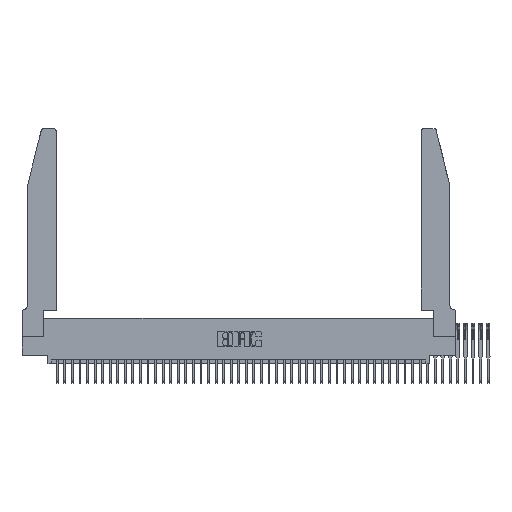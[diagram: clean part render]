
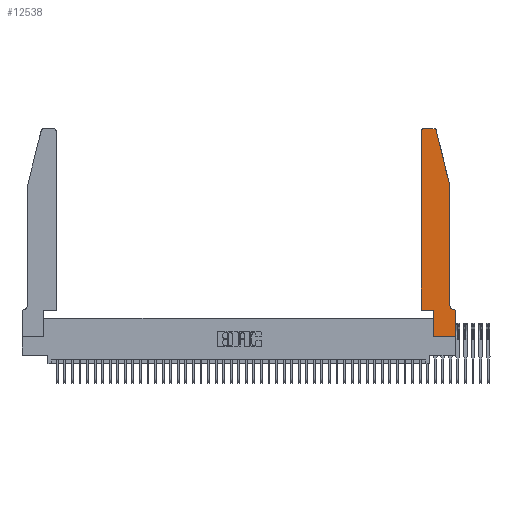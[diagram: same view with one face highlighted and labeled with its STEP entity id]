
A CAD part, top view. The second image highlights one B-rep face of the part: STEP entity #12538.
In plain terms, the highlighted face is planar.
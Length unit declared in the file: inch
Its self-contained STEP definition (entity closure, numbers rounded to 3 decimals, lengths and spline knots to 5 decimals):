
#137 = LINE ( 'NONE', #8807, #24539 ) ;
#570 = EDGE_CURVE ( 'NONE', #32551, #26741, #822, .T. ) ;
#822 = CIRCLE ( 'NONE', #26208, 0.03 ) ;
#879 = ORIENTED_EDGE ( 'NONE', *, *, #991, .F. ) ;
#991 = EDGE_CURVE ( 'NONE', #1038, #39043, #26149, .T. ) ;
#1038 = VERTEX_POINT ( 'NONE', #5005 ) ;
#1140 = LINE ( 'NONE', #37753, #32993 ) ;
#1830 = LINE ( 'NONE', #24609, #24405 ) ;
#2118 = ORIENTED_EDGE ( 'NONE', *, *, #23229, .T. ) ;
#2352 = VECTOR ( 'NONE', #24410, 39.37008 ) ;
#3321 = FACE_OUTER_BOUND ( 'NONE', #11253, .T. ) ;
#4335 = CARTESIAN_POINT ( 'NONE',  ( 0.284, 2.75, 0. ) ) ;
#4672 = CARTESIAN_POINT ( 'NONE',  ( 0.2865, 0.35, 0. ) ) ;
#4699 = ORIENTED_EDGE ( 'NONE', *, *, #27769, .F. ) ;
#5001 = VERTEX_POINT ( 'NONE', #5558 ) ;
#5005 = CARTESIAN_POINT ( 'NONE',  ( 0.2865, 0., 0. ) ) ;
#5558 = CARTESIAN_POINT ( 'NONE',  ( 0.4505, 0.35, 0. ) ) ;
#5604 = CARTESIAN_POINT ( 'NONE',  ( 0.4505, 0.35, 0. ) ) ;
#5774 = EDGE_CURVE ( 'NONE', #5001, #26741, #22489, .T. ) ;
#5792 = ORIENTED_EDGE ( 'NONE', *, *, #22735, .F. ) ;
#6070 = CARTESIAN_POINT ( 'NONE',  ( 0., 0.35, 0. ) ) ;
#6268 = VECTOR ( 'NONE', #22689, 39.37008 ) ;
#8549 = CARTESIAN_POINT ( 'NONE',  ( 0.0755, 0.35, 0. ) ) ;
#8642 = CIRCLE ( 'NONE', #31758, 0.07 ) ;
#8807 = CARTESIAN_POINT ( 'NONE',  ( 0.2605, 2.75, 0. ) ) ;
#8906 = CARTESIAN_POINT ( 'NONE',  ( 0.4205, 2.72, 0. ) ) ;
#9178 = EDGE_CURVE ( 'NONE', #17915, #32326, #27027, .T. ) ;
#9255 = DIRECTION ( 'NONE',  ( 1., 0., 0. ) ) ;
#9429 = EDGE_CURVE ( 'NONE', #32326, #1038, #1140, .T. ) ;
#9470 = ORIENTED_EDGE ( 'NONE', *, *, #16311, .F. ) ;
#9725 = CARTESIAN_POINT ( 'NONE',  ( 0., 0.35, 0. ) ) ;
#10323 = CARTESIAN_POINT ( 'NONE',  ( 0.0755, 0.42, 0. ) ) ;
#10536 = VECTOR ( 'NONE', #24941, 39.37008 ) ;
#11116 = CARTESIAN_POINT ( 'NONE',  ( 0.2865, 0.35, 0. ) ) ;
#11253 = EDGE_LOOP ( 'NONE', ( #5792, #2118, #29551, #14066, #12276, #9470, #879, #33978, #34165, #29420, #4699, #33963 ) ) ;
#12011 = DIRECTION ( 'NONE',  ( 0., 1., 0. ) ) ;
#12122 = DIRECTION ( 'NONE',  ( 1., 0., 0. ) ) ;
#12276 = ORIENTED_EDGE ( 'NONE', *, *, #5774, .F. ) ;
#12538 = ADVANCED_FACE ( 'NONE', ( #3321 ), #37759, .F. ) ;
#13747 = CARTESIAN_POINT ( 'NONE',  ( 0.4205, 2.75, 0. ) ) ;
#14066 = ORIENTED_EDGE ( 'NONE', *, *, #570, .T. ) ;
#15703 = EDGE_CURVE ( 'NONE', #26108, #30492, #35897, .T. ) ;
#15738 = CARTESIAN_POINT ( 'NONE',  ( 0.4505, 2.72, 0. ) ) ;
#16311 = EDGE_CURVE ( 'NONE', #39043, #5001, #1830, .T. ) ;
#17507 = VERTEX_POINT ( 'NONE', #4335 ) ;
#17626 = CARTESIAN_POINT ( 'NONE',  ( 0.0055, 0.42, 0. ) ) ;
#17915 = VERTEX_POINT ( 'NONE', #9725 ) ;
#18543 = CARTESIAN_POINT ( 'NONE',  ( 0.0755, 2., 0. ) ) ;
#18570 = VECTOR ( 'NONE', #39979, 39.37008 ) ;
#18645 = CARTESIAN_POINT ( 'NONE',  ( 0.284, 2.72, 0. ) ) ;
#19512 = CARTESIAN_POINT ( 'NONE',  ( 0.0755, 2., 0. ) ) ;
#20811 = DIRECTION ( 'NONE',  ( -1., 0., 0. ) ) ;
#21139 = CIRCLE ( 'NONE', #39325, 0.03 ) ;
#21815 = CARTESIAN_POINT ( 'NONE',  ( 0.25487, 2.72718, 0. ) ) ;
#21828 = DIRECTION ( 'NONE',  ( 1., 0., 0. ) ) ;
#22489 = LINE ( 'NONE', #5604, #38421 ) ;
#22689 = DIRECTION ( 'NONE',  ( -0.239, -0.971, 0. ) ) ;
#22735 = EDGE_CURVE ( 'NONE', #38230, #26108, #23180, .T. ) ;
#23180 = LINE ( 'NONE', #19512, #6268 ) ;
#23229 = EDGE_CURVE ( 'NONE', #38230, #17507, #21139, .T. ) ;
#24405 = VECTOR ( 'NONE', #27830, 39.37008 ) ;
#24410 = DIRECTION ( 'NONE',  ( -1., 0., 0. ) ) ;
#24539 = VECTOR ( 'NONE', #31067, 39.37008 ) ;
#24609 = CARTESIAN_POINT ( 'NONE',  ( 0.4505, 0.35, 0. ) ) ;
#24941 = DIRECTION ( 'NONE',  ( 0., -1., 0. ) ) ;
#25162 = VECTOR ( 'NONE', #26953, 39.37008 ) ;
#26108 = VERTEX_POINT ( 'NONE', #40931 ) ;
#26149 = LINE ( 'NONE', #11116, #25162 ) ;
#26208 = AXIS2_PLACEMENT_3D ( 'NONE', #8906, #31181, #12122 ) ;
#26741 = VERTEX_POINT ( 'NONE', #15738 ) ;
#26953 = DIRECTION ( 'NONE',  ( 0., 1., 0. ) ) ;
#27027 = LINE ( 'NONE', #30422, #18570 ) ;
#27743 = LINE ( 'NONE', #8549, #2352 ) ;
#27769 = EDGE_CURVE ( 'NONE', #30492, #40398, #8642, .T. ) ;
#27830 = DIRECTION ( 'NONE',  ( 1., 0., 0. ) ) ;
#28325 = DIRECTION ( 'NONE',  ( 0., 0., 1. ) ) ;
#28546 = AXIS2_PLACEMENT_3D ( 'NONE', #6070, #28325, #9255 ) ;
#29420 = ORIENTED_EDGE ( 'NONE', *, *, #36470, .F. ) ;
#29551 = ORIENTED_EDGE ( 'NONE', *, *, #41181, .F. ) ;
#30422 = CARTESIAN_POINT ( 'NONE',  ( 0., 0., 0. ) ) ;
#30492 = VERTEX_POINT ( 'NONE', #10323 ) ;
#31067 = DIRECTION ( 'NONE',  ( -1., 0., 0. ) ) ;
#31181 = DIRECTION ( 'NONE',  ( 0., 0., -1. ) ) ;
#31758 = AXIS2_PLACEMENT_3D ( 'NONE', #17626, #39837, #20811 ) ;
#32326 = VERTEX_POINT ( 'NONE', #41131 ) ;
#32551 = VERTEX_POINT ( 'NONE', #13747 ) ;
#32993 = VECTOR ( 'NONE', #37894, 39.37008 ) ;
#33963 = ORIENTED_EDGE ( 'NONE', *, *, #15703, .F. ) ;
#33978 = ORIENTED_EDGE ( 'NONE', *, *, #9429, .F. ) ;
#34165 = ORIENTED_EDGE ( 'NONE', *, *, #9178, .F. ) ;
#35897 = LINE ( 'NONE', #18543, #10536 ) ;
#36470 = EDGE_CURVE ( 'NONE', #40398, #17915, #27743, .T. ) ;
#37753 = CARTESIAN_POINT ( 'NONE',  ( 0., 0., 0. ) ) ;
#37759 = PLANE ( 'NONE',  #28546 ) ;
#37894 = DIRECTION ( 'NONE',  ( 1., 0., 0. ) ) ;
#38230 = VERTEX_POINT ( 'NONE', #21815 ) ;
#38421 = VECTOR ( 'NONE', #12011, 39.37008 ) ;
#39043 = VERTEX_POINT ( 'NONE', #4672 ) ;
#39294 = CARTESIAN_POINT ( 'NONE',  ( 0.0055, 0.35, 0. ) ) ;
#39325 = AXIS2_PLACEMENT_3D ( 'NONE', #18645, #40866, #21828 ) ;
#39837 = DIRECTION ( 'NONE',  ( 0., 0., -1. ) ) ;
#39979 = DIRECTION ( 'NONE',  ( 0., -1., 0. ) ) ;
#40398 = VERTEX_POINT ( 'NONE', #39294 ) ;
#40866 = DIRECTION ( 'NONE',  ( 0., 0., -1. ) ) ;
#40931 = CARTESIAN_POINT ( 'NONE',  ( 0.0755, 2., 0. ) ) ;
#41131 = CARTESIAN_POINT ( 'NONE',  ( 0., 0., 0. ) ) ;
#41181 = EDGE_CURVE ( 'NONE', #32551, #17507, #137, .T. ) ;
